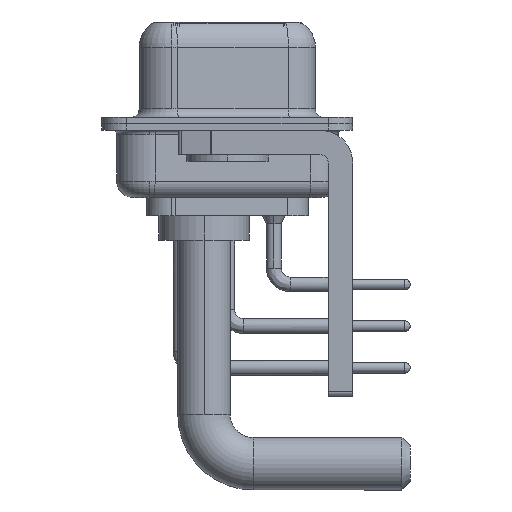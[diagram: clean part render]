
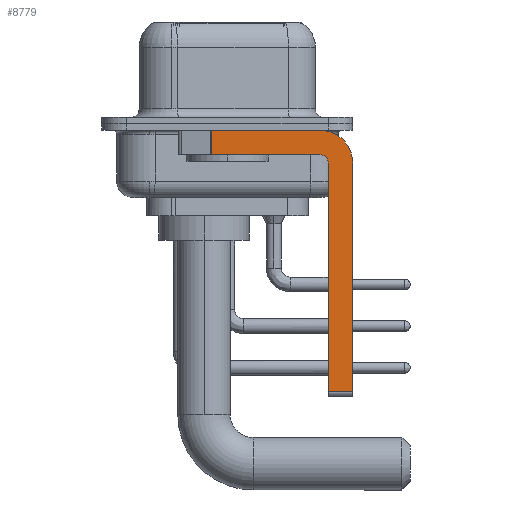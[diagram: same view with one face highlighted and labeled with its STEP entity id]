
A CAD part, left-side view. The second image highlights one B-rep face of the part: STEP entity #8779.
In plain terms, the highlighted planar face has unit normal (-1, 0, 0).
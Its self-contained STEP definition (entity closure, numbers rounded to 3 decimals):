
#572 = LINE ( 'NONE', #11278, #26349 ) ;
#925 = DIRECTION ( 'NONE',  ( 0., -1., 0. ) ) ;
#1090 = VERTEX_POINT ( 'NONE', #28445 ) ;
#1581 = EDGE_CURVE ( 'NONE', #11537, #14650, #6483, .T. ) ;
#1606 = VERTEX_POINT ( 'NONE', #31558 ) ;
#2113 = DIRECTION ( 'NONE',  ( 0., -1., 0. ) ) ;
#2615 = VECTOR ( 'NONE', #2113, 1000. ) ;
#3368 = LINE ( 'NONE', #27758, #5114 ) ;
#3415 = CARTESIAN_POINT ( 'NONE',  ( -2.9, 0.978, -1.9 ) ) ;
#3641 = ORIENTED_EDGE ( 'NONE', *, *, #18423, .F. ) ;
#4217 = CARTESIAN_POINT ( 'NONE',  ( -2.9, -5.65, -1.9 ) ) ;
#4263 = PLANE ( 'NONE',  #29763 ) ;
#4574 = CARTESIAN_POINT ( 'NONE',  ( -2.9, 3., -0.4 ) ) ;
#5006 = ORIENTED_EDGE ( 'NONE', *, *, #1581, .F. ) ;
#5114 = VECTOR ( 'NONE', #33392, 1000. ) ;
#5145 = ORIENTED_EDGE ( 'NONE', *, *, #24955, .F. ) ;
#6483 = LINE ( 'NONE', #34031, #25990 ) ;
#6701 = DIRECTION ( 'NONE',  ( 0., 1., 0. ) ) ;
#6738 = CARTESIAN_POINT ( 'NONE',  ( -2.9, 0.978, -0.4 ) ) ;
#7083 = FACE_OUTER_BOUND ( 'NONE', #33279, .T. ) ;
#7887 = CARTESIAN_POINT ( 'NONE',  ( -2.9, -5.65, -1.9 ) ) ;
#8779 = ADVANCED_FACE ( 'NONE', ( #7083 ), #4263, .F. ) ;
#9474 = ORIENTED_EDGE ( 'NONE', *, *, #21962, .T. ) ;
#9700 = CARTESIAN_POINT ( 'NONE',  ( -2.9, -5.65, -2.4 ) ) ;
#10143 = DIRECTION ( 'NONE',  ( 0., 0., 1. ) ) ;
#10358 = VERTEX_POINT ( 'NONE', #16544 ) ;
#10472 = EDGE_CURVE ( 'NONE', #11537, #10358, #572, .T. ) ;
#11278 = CARTESIAN_POINT ( 'NONE',  ( -2.9, -5.65, -16.35 ) ) ;
#11537 = VERTEX_POINT ( 'NONE', #15732 ) ;
#11753 = VERTEX_POINT ( 'NONE', #3415 ) ;
#14370 = DIRECTION ( 'NONE',  ( -1., 0., 0. ) ) ;
#14650 = VERTEX_POINT ( 'NONE', #16149 ) ;
#15732 = CARTESIAN_POINT ( 'NONE',  ( -2.9, -6.15, -16.35 ) ) ;
#15762 = ORIENTED_EDGE ( 'NONE', *, *, #10472, .T. ) ;
#15979 = VERTEX_POINT ( 'NONE', #6738 ) ;
#16149 = CARTESIAN_POINT ( 'NONE',  ( -2.9, -6.15, -2.4 ) ) ;
#16544 = CARTESIAN_POINT ( 'NONE',  ( -2.9, -7.65, -16.35 ) ) ;
#17567 = LINE ( 'NONE', #4217, #20521 ) ;
#18423 = EDGE_CURVE ( 'NONE', #1606, #10358, #18761, .T. ) ;
#18434 = VERTEX_POINT ( 'NONE', #7887 ) ;
#18488 = DIRECTION ( 'NONE',  ( 0., 0., -1. ) ) ;
#18536 = EDGE_CURVE ( 'NONE', #14650, #18434, #28400, .T. ) ;
#18761 = LINE ( 'NONE', #23862, #25022 ) ;
#20521 = VECTOR ( 'NONE', #6701, 1000. ) ;
#20992 = CIRCLE ( 'NONE', #28839, 2. ) ;
#21962 = EDGE_CURVE ( 'NONE', #15979, #11753, #3368, .T. ) ;
#23582 = CARTESIAN_POINT ( 'NONE',  ( -2.9, -5.65, -2.4 ) ) ;
#23862 = CARTESIAN_POINT ( 'NONE',  ( -2.9, -7.65, -2.4 ) ) ;
#24955 = EDGE_CURVE ( 'NONE', #1090, #1606, #20992, .T. ) ;
#25022 = VECTOR ( 'NONE', #34404, 1000. ) ;
#25103 = ORIENTED_EDGE ( 'NONE', *, *, #28006, .F. ) ;
#25990 = VECTOR ( 'NONE', #10143, 1000. ) ;
#26166 = AXIS2_PLACEMENT_3D ( 'NONE', #30690, #14370, #32986 ) ;
#26349 = VECTOR ( 'NONE', #925, 1000. ) ;
#27758 = CARTESIAN_POINT ( 'NONE',  ( -2.9, 0.978, -1.9 ) ) ;
#28006 = EDGE_CURVE ( 'NONE', #18434, #11753, #17567, .T. ) ;
#28400 = CIRCLE ( 'NONE', #26166, 0.5 ) ;
#28445 = CARTESIAN_POINT ( 'NONE',  ( -2.9, -5.65, -0.4 ) ) ;
#28839 = AXIS2_PLACEMENT_3D ( 'NONE', #23582, #32013, #18488 ) ;
#29763 = AXIS2_PLACEMENT_3D ( 'NONE', #9700, #31297, #34282 ) ;
#30550 = ORIENTED_EDGE ( 'NONE', *, *, #18536, .F. ) ;
#30690 = CARTESIAN_POINT ( 'NONE',  ( -2.9, -5.65, -2.4 ) ) ;
#31297 = DIRECTION ( 'NONE',  ( 1., 0., 0. ) ) ;
#31558 = CARTESIAN_POINT ( 'NONE',  ( -2.9, -7.65, -2.4 ) ) ;
#32013 = DIRECTION ( 'NONE',  ( 1., 0., 0. ) ) ;
#32986 = DIRECTION ( 'NONE',  ( 0., 0., 1. ) ) ;
#33023 = ORIENTED_EDGE ( 'NONE', *, *, #34668, .F. ) ;
#33279 = EDGE_LOOP ( 'NONE', ( #33023, #9474, #25103, #30550, #5006, #15762, #3641, #5145 ) ) ;
#33392 = DIRECTION ( 'NONE',  ( 0., 0., -1. ) ) ;
#34031 = CARTESIAN_POINT ( 'NONE',  ( -2.9, -6.15, -16.6 ) ) ;
#34282 = DIRECTION ( 'NONE',  ( 0., 0., -1. ) ) ;
#34404 = DIRECTION ( 'NONE',  ( 0., 0., -1. ) ) ;
#34429 = LINE ( 'NONE', #4574, #2615 ) ;
#34668 = EDGE_CURVE ( 'NONE', #15979, #1090, #34429, .T. ) ;
